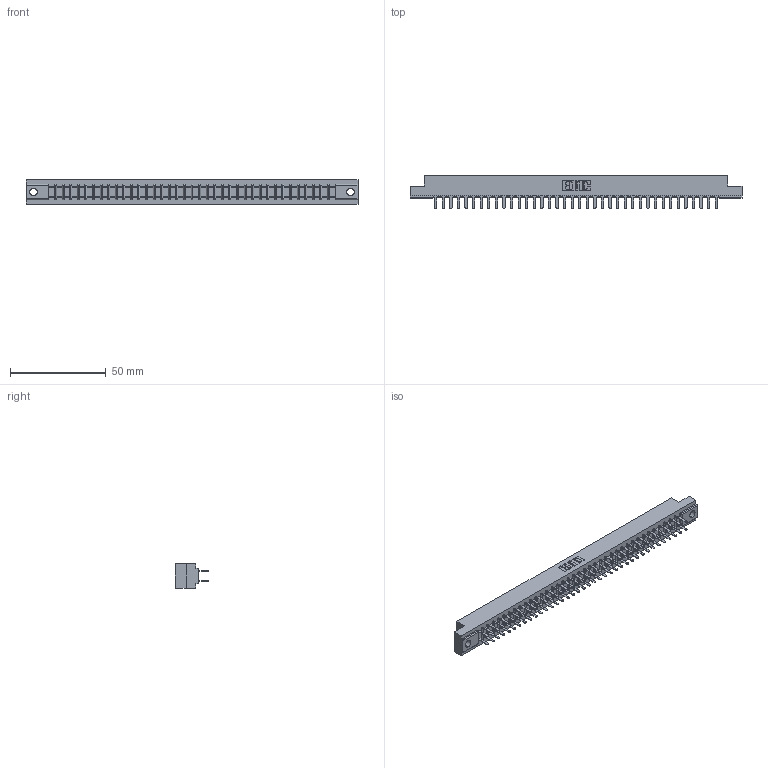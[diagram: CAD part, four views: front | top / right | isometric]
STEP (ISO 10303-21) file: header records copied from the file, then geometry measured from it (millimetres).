
FILE_DESCRIPTION (( 'STEP AP203' ), '1' );
FILE_NAME ('357-076-520-202.STEP', '2018-08-12T21:13:55', ( '' ), ( '' ), 'SwSTEP 2.0', 'SolidWorks 2016', '' );
FILE_SCHEMA (( 'CONFIG_CONTROL_DESIGN' ));
Length unit declared in the file: inch
Products named in the file (3): 307 Part_.128 Dia Mounting Holes; 307-290-001_520; 357-076-520-202
Assembly tree (77 placements, depth 2):
  357-076-520-202
    307 Part_.128 Dia Mounting Holes
    307-290-001_520  x76
Bounding box: 173.58 x 17.42 x 12.7 mm (x, y, z)
Volume: 18398.1 mm3; surface area: 22354.1 mm2
Topology: 77 solids, 77 shells, 3653 faces, 10203 edges, 6594 vertices
Faces by surface type: plane 2426, cylinder 1149, sphere 78
Entity records: 34256 total; most frequent: CARTESIAN_POINT 5602, ORIENTED_EDGE 5550, DIRECTION 5489, EDGE_CURVE 2775, LINE 2127, VECTOR 2127, VERTEX_POINT 1794, AXIS2_PLACEMENT_3D 1681
